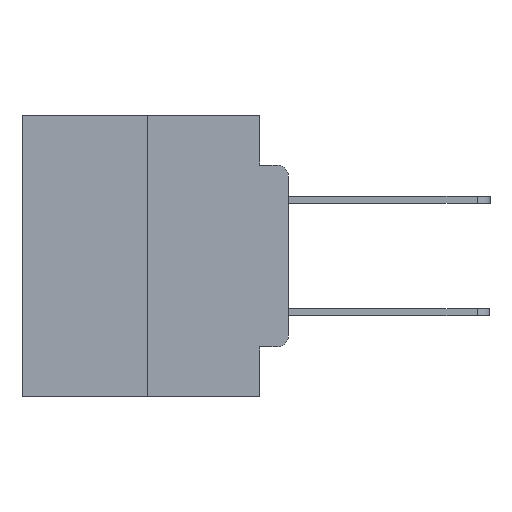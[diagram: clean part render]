
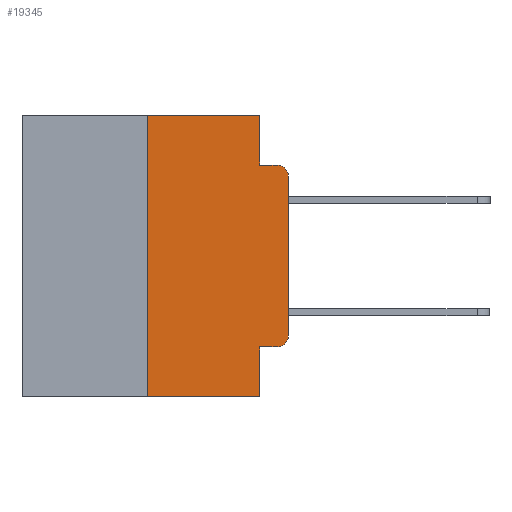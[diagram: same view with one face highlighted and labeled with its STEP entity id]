
A CAD part, left-side view. The second image highlights one B-rep face of the part: STEP entity #19345.
In plain terms, the highlighted planar face has unit normal (-1, 0, 0).
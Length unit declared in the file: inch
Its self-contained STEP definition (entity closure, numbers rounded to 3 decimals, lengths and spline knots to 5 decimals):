
#63 = VERTEX_POINT ( 'NONE', #23590 ) ;
#521 = EDGE_CURVE ( 'NONE', #7666, #1162, #3499, .T. ) ;
#657 = CARTESIAN_POINT ( 'NONE',  ( 0., 0.051, -0.5 ) ) ;
#853 = CARTESIAN_POINT ( 'NONE',  ( 0., 0.051, 0. ) ) ;
#1162 = VERTEX_POINT ( 'NONE', #8655 ) ;
#1505 = AXIS2_PLACEMENT_3D ( 'NONE', #10672, #24953, #12732 ) ;
#1726 = VECTOR ( 'NONE', #17544, 39.37008 ) ;
#1829 = ORIENTED_EDGE ( 'NONE', *, *, #1910, .T. ) ;
#1910 = EDGE_CURVE ( 'NONE', #4172, #7666, #23409, .T. ) ;
#2150 = LINE ( 'NONE', #3088, #18066 ) ;
#2228 = LINE ( 'NONE', #19659, #18143 ) ;
#2241 = CARTESIAN_POINT ( 'NONE',  ( 0., 0.02, -0.3915 ) ) ;
#2491 = ORIENTED_EDGE ( 'NONE', *, *, #521, .T. ) ;
#2679 = ORIENTED_EDGE ( 'NONE', *, *, #25855, .F. ) ;
#2913 = ORIENTED_EDGE ( 'NONE', *, *, #24496, .F. ) ;
#2931 = DIRECTION ( 'NONE',  ( 0., 0., -1. ) ) ;
#3062 = ORIENTED_EDGE ( 'NONE', *, *, #10173, .F. ) ;
#3088 = CARTESIAN_POINT ( 'NONE',  ( 0., 0.473, -0.5 ) ) ;
#3112 = ORIENTED_EDGE ( 'NONE', *, *, #12172, .F. ) ;
#3222 = ORIENTED_EDGE ( 'NONE', *, *, #26186, .T. ) ;
#3303 = ORIENTED_EDGE ( 'NONE', *, *, #5260, .F. ) ;
#3499 = CIRCLE ( 'NONE', #13183, 0.02 ) ;
#3560 = DIRECTION ( 'NONE',  ( 0., 0., 1. ) ) ;
#3646 = ORIENTED_EDGE ( 'NONE', *, *, #24986, .T. ) ;
#3767 = ORIENTED_EDGE ( 'NONE', *, *, #23669, .T. ) ;
#3939 = FACE_OUTER_BOUND ( 'NONE', #9237, .T. ) ;
#4172 = VERTEX_POINT ( 'NONE', #14345 ) ;
#4356 = DIRECTION ( 'NONE',  ( 0., 0., -1. ) ) ;
#4396 = PLANE ( 'NONE',  #1505 ) ;
#5146 = CARTESIAN_POINT ( 'NONE',  ( 0., 0.473, 0. ) ) ;
#5260 = EDGE_CURVE ( 'NONE', #16940, #26080, #2228, .T. ) ;
#5694 = CARTESIAN_POINT ( 'NONE',  ( 0., 0.25, 0. ) ) ;
#5896 = LINE ( 'NONE', #17470, #15562 ) ;
#7314 = LINE ( 'NONE', #5146, #1726 ) ;
#7666 = VERTEX_POINT ( 'NONE', #21597 ) ;
#8272 = CARTESIAN_POINT ( 'NONE',  ( 0., 0.051, -0.4115 ) ) ;
#8655 = CARTESIAN_POINT ( 'NONE',  ( 0., 0.02, -0.0885 ) ) ;
#8895 = CARTESIAN_POINT ( 'NONE',  ( 0., 0.051, -0.0885 ) ) ;
#9237 = EDGE_LOOP ( 'NONE', ( #1829, #2491, #2679, #2913, #3062, #3112, #3222, #3303, #3646, #3767 ) ) ;
#9254 = VECTOR ( 'NONE', #3560, 39.37008 ) ;
#10035 = CIRCLE ( 'NONE', #25023, 0.02 ) ;
#10173 = EDGE_CURVE ( 'NONE', #10917, #12116, #7314, .T. ) ;
#10536 = LINE ( 'NONE', #5694, #9254 ) ;
#10661 = LINE ( 'NONE', #12450, #20366 ) ;
#10672 = CARTESIAN_POINT ( 'NONE',  ( 0., 0.473, 0. ) ) ;
#10917 = VERTEX_POINT ( 'NONE', #17746 ) ;
#11369 = VERTEX_POINT ( 'NONE', #8895 ) ;
#12116 = VERTEX_POINT ( 'NONE', #21478 ) ;
#12172 = EDGE_CURVE ( 'NONE', #63, #10917, #10536, .T. ) ;
#12450 = CARTESIAN_POINT ( 'NONE',  ( 0., 0.051, -0.0885 ) ) ;
#12732 = DIRECTION ( 'NONE',  ( 0., 0., -1. ) ) ;
#13183 = AXIS2_PLACEMENT_3D ( 'NONE', #19686, #13631, #13568 ) ;
#13355 = CARTESIAN_POINT ( 'NONE',  ( 0., 0., 0. ) ) ;
#13483 = DIRECTION ( 'NONE',  ( 0., -1., 0. ) ) ;
#13484 = DIRECTION ( 'NONE',  ( 0., 0., -1. ) ) ;
#13568 = DIRECTION ( 'NONE',  ( 0., 0., -1. ) ) ;
#13631 = DIRECTION ( 'NONE',  ( -1., 0., 0. ) ) ;
#14345 = CARTESIAN_POINT ( 'NONE',  ( 0., 0., -0.3915 ) ) ;
#14525 = DIRECTION ( 'NONE',  ( 0., -1., 0. ) ) ;
#15562 = VECTOR ( 'NONE', #19571, 39.37008 ) ;
#15869 = VECTOR ( 'NONE', #2931, 39.37008 ) ;
#16260 = VERTEX_POINT ( 'NONE', #22575 ) ;
#16761 = DIRECTION ( 'NONE',  ( -1., 0., 0. ) ) ;
#16940 = VERTEX_POINT ( 'NONE', #8272 ) ;
#17470 = CARTESIAN_POINT ( 'NONE',  ( 0., 0.051, -0.4115 ) ) ;
#17544 = DIRECTION ( 'NONE',  ( 0., -1., 0. ) ) ;
#17746 = CARTESIAN_POINT ( 'NONE',  ( 0., 0.25, 0. ) ) ;
#18011 = VECTOR ( 'NONE', #21053, 39.37008 ) ;
#18066 = VECTOR ( 'NONE', #13483, 39.37008 ) ;
#18143 = VECTOR ( 'NONE', #13484, 39.37008 ) ;
#19345 = ADVANCED_FACE ( 'NONE', ( #3939 ), #4396, .F. ) ;
#19571 = DIRECTION ( 'NONE',  ( 0., -1., 0. ) ) ;
#19659 = CARTESIAN_POINT ( 'NONE',  ( 0., 0.051, 0. ) ) ;
#19686 = CARTESIAN_POINT ( 'NONE',  ( 0., 0.02, -0.1085 ) ) ;
#20366 = VECTOR ( 'NONE', #14525, 39.37008 ) ;
#21053 = DIRECTION ( 'NONE',  ( 0., 0., 1. ) ) ;
#21478 = CARTESIAN_POINT ( 'NONE',  ( 0., 0.051, 0. ) ) ;
#21597 = CARTESIAN_POINT ( 'NONE',  ( 0., 0., -0.1085 ) ) ;
#21984 = LINE ( 'NONE', #853, #15869 ) ;
#22575 = CARTESIAN_POINT ( 'NONE',  ( 0., 0.02, -0.4115 ) ) ;
#23409 = LINE ( 'NONE', #13355, #18011 ) ;
#23590 = CARTESIAN_POINT ( 'NONE',  ( 0., 0.25, -0.5 ) ) ;
#23669 = EDGE_CURVE ( 'NONE', #16260, #4172, #10035, .T. ) ;
#24496 = EDGE_CURVE ( 'NONE', #12116, #11369, #21984, .T. ) ;
#24953 = DIRECTION ( 'NONE',  ( 1., 0., 0. ) ) ;
#24986 = EDGE_CURVE ( 'NONE', #16940, #16260, #5896, .T. ) ;
#25023 = AXIS2_PLACEMENT_3D ( 'NONE', #2241, #16761, #4356 ) ;
#25855 = EDGE_CURVE ( 'NONE', #11369, #1162, #10661, .T. ) ;
#26080 = VERTEX_POINT ( 'NONE', #657 ) ;
#26186 = EDGE_CURVE ( 'NONE', #63, #26080, #2150, .T. ) ;
